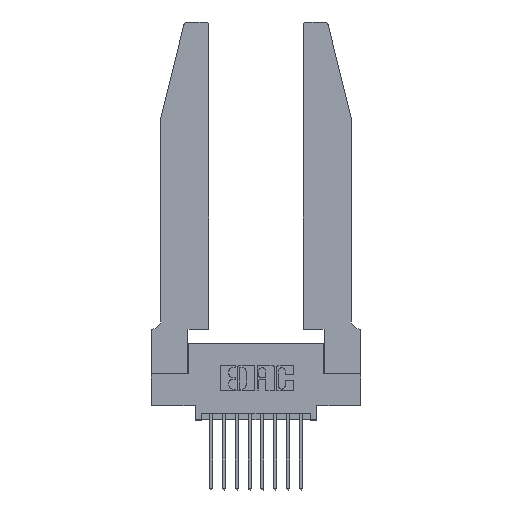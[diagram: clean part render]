
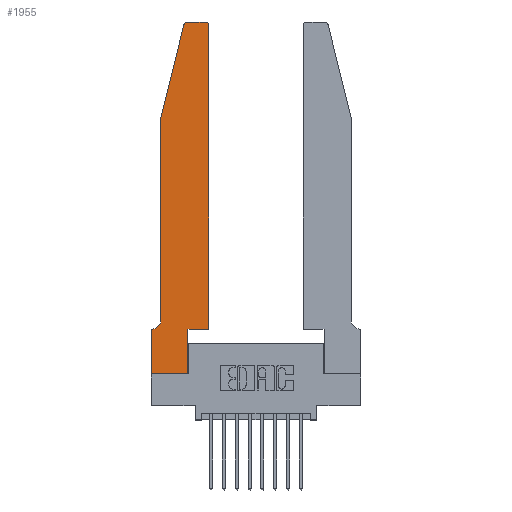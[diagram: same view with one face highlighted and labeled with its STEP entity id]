
A CAD part, top view. The second image highlights one B-rep face of the part: STEP entity #1955.
In plain terms, the highlighted planar face has unit normal (0, 0, 1).
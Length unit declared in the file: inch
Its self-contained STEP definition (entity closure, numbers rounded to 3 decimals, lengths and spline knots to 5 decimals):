
#29 = CARTESIAN_POINT ( 'NONE',  ( 0., 0.35, 0.37 ) ) ;
#101 = VERTEX_POINT ( 'NONE', #3263 ) ;
#345 = VERTEX_POINT ( 'NONE', #14420 ) ;
#410 = DIRECTION ( 'NONE',  ( 1., 0., 0. ) ) ;
#508 = VERTEX_POINT ( 'NONE', #11016 ) ;
#761 = ORIENTED_EDGE ( 'NONE', *, *, #9949, .T. ) ;
#766 = VERTEX_POINT ( 'NONE', #5358 ) ;
#845 = DIRECTION ( 'NONE',  ( -1., 0., 0. ) ) ;
#866 = DIRECTION ( 'NONE',  ( 1., 0., 0. ) ) ;
#1069 = EDGE_CURVE ( 'NONE', #101, #11257, #4412, .T. ) ;
#1127 = VECTOR ( 'NONE', #12181, 39.37008 ) ;
#1148 = VECTOR ( 'NONE', #6800, 39.37008 ) ;
#1418 = DIRECTION ( 'NONE',  ( 0., 0., -1. ) ) ;
#1468 = VECTOR ( 'NONE', #8350, 39.37008 ) ;
#1656 = CIRCLE ( 'NONE', #2202, 0.03 ) ;
#1865 = LINE ( 'NONE', #4670, #7916 ) ;
#1955 = ADVANCED_FACE ( 'NONE', ( #12320 ), #8290, .T. ) ;
#2125 = CARTESIAN_POINT ( 'NONE',  ( 0.25487, 2.72718, 0.37 ) ) ;
#2202 = AXIS2_PLACEMENT_3D ( 'NONE', #15426, #8128, #866 ) ;
#2369 = DIRECTION ( 'NONE',  ( -1., 0., 0. ) ) ;
#2559 = EDGE_CURVE ( 'NONE', #13799, #6816, #10787, .T. ) ;
#2666 = ORIENTED_EDGE ( 'NONE', *, *, #5031, .T. ) ;
#3263 = CARTESIAN_POINT ( 'NONE',  ( 0.2865, 0.35, 0.37 ) ) ;
#3297 = ORIENTED_EDGE ( 'NONE', *, *, #14531, .T. ) ;
#3464 = CARTESIAN_POINT ( 'NONE',  ( 0.4205, 2.75, 0.37 ) ) ;
#3559 = ORIENTED_EDGE ( 'NONE', *, *, #12779, .T. ) ;
#3721 = CARTESIAN_POINT ( 'NONE',  ( 0.0755, 2., 0.37 ) ) ;
#4412 = LINE ( 'NONE', #11155, #1148 ) ;
#4669 = VERTEX_POINT ( 'NONE', #2125 ) ;
#4670 = CARTESIAN_POINT ( 'NONE',  ( 0.2865, 0.35, 0.37 ) ) ;
#4710 = CARTESIAN_POINT ( 'NONE',  ( 0.0755, 2., 0.37 ) ) ;
#4766 = EDGE_CURVE ( 'NONE', #6816, #101, #1865, .T. ) ;
#4769 = EDGE_CURVE ( 'NONE', #8830, #13799, #11122, .T. ) ;
#4910 = LINE ( 'NONE', #3721, #11301 ) ;
#4948 = DIRECTION ( 'NONE',  ( 0., -1., 0. ) ) ;
#5031 = EDGE_CURVE ( 'NONE', #11257, #345, #8463, .T. ) ;
#5053 = EDGE_CURVE ( 'NONE', #13603, #4669, #1656, .T. ) ;
#5358 = CARTESIAN_POINT ( 'NONE',  ( 0.0055, 0.35, 0.37 ) ) ;
#5404 = VECTOR ( 'NONE', #14387, 39.37008 ) ;
#5423 = DIRECTION ( 'NONE',  ( 0., 0., 1. ) ) ;
#5472 = EDGE_CURVE ( 'NONE', #345, #15770, #11280, .T. ) ;
#5656 = DIRECTION ( 'NONE',  ( 0., 1., 0. ) ) ;
#5749 = CARTESIAN_POINT ( 'NONE',  ( 0., 0.35, 0.37 ) ) ;
#6800 = DIRECTION ( 'NONE',  ( 1., 0., 0. ) ) ;
#6816 = VERTEX_POINT ( 'NONE', #7079 ) ;
#7079 = CARTESIAN_POINT ( 'NONE',  ( 0.2865, 0., 0.37 ) ) ;
#7136 = DIRECTION ( 'NONE',  ( 0., 1., 0. ) ) ;
#7376 = CARTESIAN_POINT ( 'NONE',  ( 0.0755, 2., 0.37 ) ) ;
#7549 = ORIENTED_EDGE ( 'NONE', *, *, #12316, .T. ) ;
#7565 = VECTOR ( 'NONE', #845, 39.37008 ) ;
#7587 = AXIS2_PLACEMENT_3D ( 'NONE', #12651, #5423, #13882 ) ;
#7916 = VECTOR ( 'NONE', #7136, 39.37008 ) ;
#7943 = LINE ( 'NONE', #12907, #7565 ) ;
#8128 = DIRECTION ( 'NONE',  ( 0., 0., 1. ) ) ;
#8290 = PLANE ( 'NONE',  #11475 ) ;
#8350 = DIRECTION ( 'NONE',  ( 0., -1., 0. ) ) ;
#8463 = LINE ( 'NONE', #9219, #14539 ) ;
#8605 = LINE ( 'NONE', #4710, #5404 ) ;
#8666 = CARTESIAN_POINT ( 'NONE',  ( 0.0055, 0.42, 0.37 ) ) ;
#8761 = DIRECTION ( 'NONE',  ( 0., 0., 1. ) ) ;
#8830 = VERTEX_POINT ( 'NONE', #29 ) ;
#8898 = AXIS2_PLACEMENT_3D ( 'NONE', #8666, #1418, #9886 ) ;
#9182 = EDGE_CURVE ( 'NONE', #766, #8830, #7943, .T. ) ;
#9219 = CARTESIAN_POINT ( 'NONE',  ( 0.4505, 0.35, 0.37 ) ) ;
#9364 = ORIENTED_EDGE ( 'NONE', *, *, #5472, .T. ) ;
#9545 = CARTESIAN_POINT ( 'NONE',  ( 0., 0., 0.37 ) ) ;
#9886 = DIRECTION ( 'NONE',  ( -1., 0., 0. ) ) ;
#9949 = EDGE_CURVE ( 'NONE', #11181, #508, #4910, .T. ) ;
#10157 = ORIENTED_EDGE ( 'NONE', *, *, #9182, .T. ) ;
#10167 = ORIENTED_EDGE ( 'NONE', *, *, #5053, .T. ) ;
#10401 = ORIENTED_EDGE ( 'NONE', *, *, #1069, .T. ) ;
#10730 = CARTESIAN_POINT ( 'NONE',  ( 0., 0., 0.37 ) ) ;
#10787 = LINE ( 'NONE', #11573, #1127 ) ;
#10827 = CARTESIAN_POINT ( 'NONE',  ( 0.2605, 2.75, 0.37 ) ) ;
#11016 = CARTESIAN_POINT ( 'NONE',  ( 0.0755, 0.42, 0.37 ) ) ;
#11111 = CARTESIAN_POINT ( 'NONE',  ( 0.284, 2.75, 0.37 ) ) ;
#11122 = LINE ( 'NONE', #9545, #1468 ) ;
#11155 = CARTESIAN_POINT ( 'NONE',  ( 0.4505, 0.35, 0.37 ) ) ;
#11181 = VERTEX_POINT ( 'NONE', #7376 ) ;
#11202 = VECTOR ( 'NONE', #2369, 39.37008 ) ;
#11257 = VERTEX_POINT ( 'NONE', #12384 ) ;
#11280 = CIRCLE ( 'NONE', #7587, 0.03 ) ;
#11289 = ORIENTED_EDGE ( 'NONE', *, *, #2559, .T. ) ;
#11301 = VECTOR ( 'NONE', #4948, 39.37008 ) ;
#11475 = AXIS2_PLACEMENT_3D ( 'NONE', #5749, #8761, #410 ) ;
#11573 = CARTESIAN_POINT ( 'NONE',  ( 0., 0., 0.37 ) ) ;
#12181 = DIRECTION ( 'NONE',  ( 1., 0., 0. ) ) ;
#12316 = EDGE_CURVE ( 'NONE', #508, #766, #15093, .T. ) ;
#12320 = FACE_OUTER_BOUND ( 'NONE', #15262, .T. ) ;
#12384 = CARTESIAN_POINT ( 'NONE',  ( 0.4505, 0.35, 0.37 ) ) ;
#12651 = CARTESIAN_POINT ( 'NONE',  ( 0.4205, 2.72, 0.37 ) ) ;
#12779 = EDGE_CURVE ( 'NONE', #4669, #11181, #8605, .T. ) ;
#12907 = CARTESIAN_POINT ( 'NONE',  ( 0.0755, 0.35, 0.37 ) ) ;
#12923 = ORIENTED_EDGE ( 'NONE', *, *, #4769, .T. ) ;
#13603 = VERTEX_POINT ( 'NONE', #11111 ) ;
#13799 = VERTEX_POINT ( 'NONE', #10730 ) ;
#13818 = ORIENTED_EDGE ( 'NONE', *, *, #4766, .T. ) ;
#13882 = DIRECTION ( 'NONE',  ( 1., 0., 0. ) ) ;
#14387 = DIRECTION ( 'NONE',  ( -0.239, -0.971, 0. ) ) ;
#14420 = CARTESIAN_POINT ( 'NONE',  ( 0.4505, 2.72, 0.37 ) ) ;
#14440 = LINE ( 'NONE', #10827, #11202 ) ;
#14531 = EDGE_CURVE ( 'NONE', #15770, #13603, #14440, .T. ) ;
#14539 = VECTOR ( 'NONE', #5656, 39.37008 ) ;
#15093 = CIRCLE ( 'NONE', #8898, 0.07 ) ;
#15262 = EDGE_LOOP ( 'NONE', ( #3297, #10167, #3559, #761, #7549, #10157, #12923, #11289, #13818, #10401, #2666, #9364 ) ) ;
#15426 = CARTESIAN_POINT ( 'NONE',  ( 0.284, 2.72, 0.37 ) ) ;
#15770 = VERTEX_POINT ( 'NONE', #3464 ) ;
